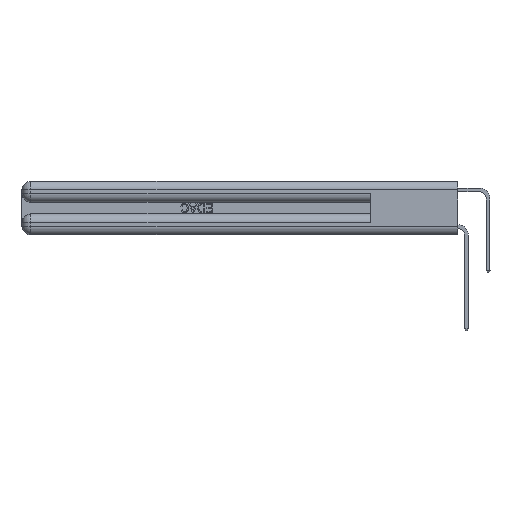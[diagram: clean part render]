
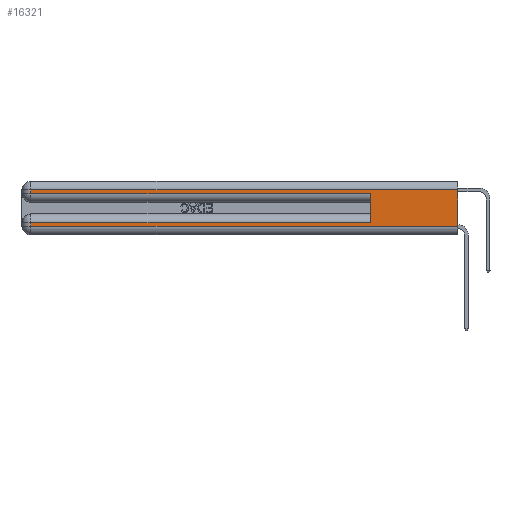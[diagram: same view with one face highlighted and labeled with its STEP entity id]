
A CAD part, left-side view. The second image highlights one B-rep face of the part: STEP entity #16321.
In plain terms, the highlighted planar face has unit normal (-1, 0, 0).
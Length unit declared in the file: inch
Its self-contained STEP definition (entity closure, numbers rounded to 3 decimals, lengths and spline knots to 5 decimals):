
#1487 = VECTOR ( 'NONE', #17132, 39.37008 ) ;
#1824 = EDGE_CURVE ( 'NONE', #18227, #11283, #36909, .T. ) ;
#1984 = DIRECTION ( 'NONE',  ( 0., 0., -1. ) ) ;
#2700 = VECTOR ( 'NONE', #9119, 39.37008 ) ;
#3379 = CARTESIAN_POINT ( 'NONE',  ( 0., 0., 0.31 ) ) ;
#3867 = DIRECTION ( 'NONE',  ( 0., 1., 0. ) ) ;
#3894 = EDGE_CURVE ( 'NONE', #21264, #23837, #12537, .T. ) ;
#4495 = CARTESIAN_POINT ( 'NONE',  ( 0., 0.6, 0.145 ) ) ;
#4929 = CARTESIAN_POINT ( 'NONE',  ( 0., 2.94, 0.285 ) ) ;
#5241 = CARTESIAN_POINT ( 'NONE',  ( 0., 2.94, 0.37 ) ) ;
#5572 = LINE ( 'NONE', #29467, #17856 ) ;
#6898 = CARTESIAN_POINT ( 'NONE',  ( 0., 0., 0.085 ) ) ;
#7422 = ORIENTED_EDGE ( 'NONE', *, *, #8036, .T. ) ;
#8036 = EDGE_CURVE ( 'NONE', #38573, #10109, #18162, .T. ) ;
#9119 = DIRECTION ( 'NONE',  ( 0., -1., 0. ) ) ;
#9463 = VECTOR ( 'NONE', #18944, 39.37008 ) ;
#10096 = EDGE_CURVE ( 'NONE', #23837, #38573, #5572, .T. ) ;
#10109 = VERTEX_POINT ( 'NONE', #22961 ) ;
#10180 = VERTEX_POINT ( 'NONE', #14836 ) ;
#10435 = VECTOR ( 'NONE', #17285, 39.37008 ) ;
#11283 = VERTEX_POINT ( 'NONE', #18860 ) ;
#12537 = LINE ( 'NONE', #15895, #27286 ) ;
#12835 = EDGE_CURVE ( 'NONE', #21264, #10180, #19002, .T. ) ;
#13170 = VECTOR ( 'NONE', #31255, 39.37008 ) ;
#13183 = EDGE_LOOP ( 'NONE', ( #25599, #15460, #17073, #7422, #31292, #16371, #27673, #36081 ) ) ;
#14836 = CARTESIAN_POINT ( 'NONE',  ( 0., 0., 0.06 ) ) ;
#15460 = ORIENTED_EDGE ( 'NONE', *, *, #3894, .T. ) ;
#15758 = CARTESIAN_POINT ( 'NONE',  ( 0., 0., 0.285 ) ) ;
#15895 = CARTESIAN_POINT ( 'NONE',  ( 0., 0., 0.31 ) ) ;
#16321 = ADVANCED_FACE ( 'NONE', ( #29199 ), #29395, .F. ) ;
#16371 = ORIENTED_EDGE ( 'NONE', *, *, #1824, .T. ) ;
#16437 = CARTESIAN_POINT ( 'NONE',  ( 0., 0., 0.37 ) ) ;
#17073 = ORIENTED_EDGE ( 'NONE', *, *, #10096, .T. ) ;
#17132 = DIRECTION ( 'NONE',  ( 0., 0., 1. ) ) ;
#17285 = DIRECTION ( 'NONE',  ( 0., 0., -1. ) ) ;
#17417 = VERTEX_POINT ( 'NONE', #38459 ) ;
#17562 = CARTESIAN_POINT ( 'NONE',  ( 0., 0., 0.37 ) ) ;
#17856 = VECTOR ( 'NONE', #29655, 39.37008 ) ;
#18162 = LINE ( 'NONE', #15758, #38210 ) ;
#18227 = VERTEX_POINT ( 'NONE', #31834 ) ;
#18230 = CARTESIAN_POINT ( 'NONE',  ( 0., 2.94, 0.31 ) ) ;
#18860 = CARTESIAN_POINT ( 'NONE',  ( 0., 2.94, 0.085 ) ) ;
#18944 = DIRECTION ( 'NONE',  ( 0., 1., 0. ) ) ;
#19002 = LINE ( 'NONE', #16437, #13170 ) ;
#20259 = EDGE_CURVE ( 'NONE', #18227, #10109, #37652, .T. ) ;
#20332 = DIRECTION ( 'NONE',  ( 1., 0., 0. ) ) ;
#21264 = VERTEX_POINT ( 'NONE', #3379 ) ;
#22961 = CARTESIAN_POINT ( 'NONE',  ( 0., 0.6, 0.285 ) ) ;
#23011 = LINE ( 'NONE', #5241, #10435 ) ;
#23837 = VERTEX_POINT ( 'NONE', #18230 ) ;
#24835 = EDGE_CURVE ( 'NONE', #11283, #17417, #23011, .T. ) ;
#24905 = LINE ( 'NONE', #36179, #2700 ) ;
#25599 = ORIENTED_EDGE ( 'NONE', *, *, #12835, .F. ) ;
#27286 = VECTOR ( 'NONE', #3867, 39.37008 ) ;
#27673 = ORIENTED_EDGE ( 'NONE', *, *, #24835, .T. ) ;
#29199 = FACE_OUTER_BOUND ( 'NONE', #13183, .T. ) ;
#29395 = PLANE ( 'NONE',  #37304 ) ;
#29467 = CARTESIAN_POINT ( 'NONE',  ( 0., 2.94, 0.37 ) ) ;
#29655 = DIRECTION ( 'NONE',  ( 0., 0., -1. ) ) ;
#31255 = DIRECTION ( 'NONE',  ( 0., 0., -1. ) ) ;
#31292 = ORIENTED_EDGE ( 'NONE', *, *, #20259, .F. ) ;
#31834 = CARTESIAN_POINT ( 'NONE',  ( 0., 0.6, 0.085 ) ) ;
#33543 = DIRECTION ( 'NONE',  ( 0., -1., 0. ) ) ;
#36081 = ORIENTED_EDGE ( 'NONE', *, *, #37033, .T. ) ;
#36179 = CARTESIAN_POINT ( 'NONE',  ( 0., 0., 0.06 ) ) ;
#36909 = LINE ( 'NONE', #6898, #9463 ) ;
#37033 = EDGE_CURVE ( 'NONE', #17417, #10180, #24905, .T. ) ;
#37304 = AXIS2_PLACEMENT_3D ( 'NONE', #17562, #20332, #1984 ) ;
#37652 = LINE ( 'NONE', #4495, #1487 ) ;
#38210 = VECTOR ( 'NONE', #33543, 39.37008 ) ;
#38459 = CARTESIAN_POINT ( 'NONE',  ( 0., 2.94, 0.06 ) ) ;
#38573 = VERTEX_POINT ( 'NONE', #4929 ) ;
